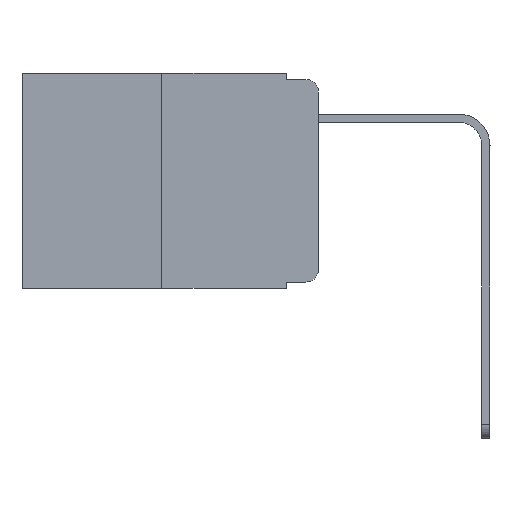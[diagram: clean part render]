
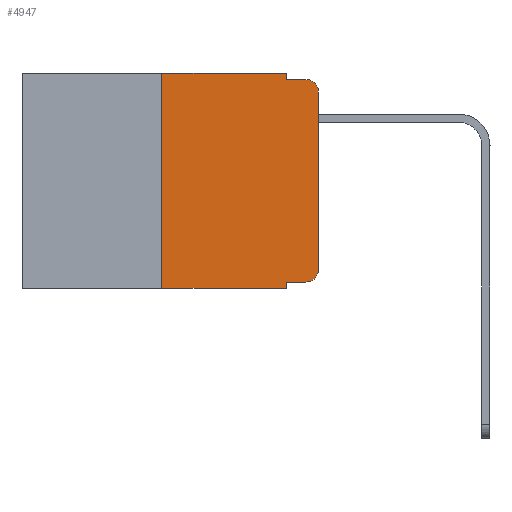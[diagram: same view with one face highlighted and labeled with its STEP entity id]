
A CAD part, left-side view. The second image highlights one B-rep face of the part: STEP entity #4947.
In plain terms, the highlighted planar face has unit normal (-1, 0, 0).
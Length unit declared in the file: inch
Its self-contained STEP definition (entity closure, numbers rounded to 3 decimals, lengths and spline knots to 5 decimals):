
#30 = VERTEX_POINT ( 'NONE', #19579 ) ;
#801 = CARTESIAN_POINT ( 'NONE',  ( 0., 0.051, -0.333 ) ) ;
#967 = ORIENTED_EDGE ( 'NONE', *, *, #7947, .F. ) ;
#1071 = VERTEX_POINT ( 'NONE', #11649 ) ;
#1330 = CARTESIAN_POINT ( 'NONE',  ( 0., 0., 0. ) ) ;
#1448 = AXIS2_PLACEMENT_3D ( 'NONE', #19015, #6102, #14162 ) ;
#1771 = VECTOR ( 'NONE', #10370, 39.37008 ) ;
#2011 = CARTESIAN_POINT ( 'NONE',  ( 0., 0.051, 0. ) ) ;
#2374 = VERTEX_POINT ( 'NONE', #12244 ) ;
#2958 = FACE_OUTER_BOUND ( 'NONE', #16848, .T. ) ;
#3194 = EDGE_CURVE ( 'NONE', #20260, #2374, #9029, .T. ) ;
#3876 = DIRECTION ( 'NONE',  ( 0., 0., -1. ) ) ;
#3958 = VECTOR ( 'NONE', #20413, 39.37008 ) ;
#4619 = ORIENTED_EDGE ( 'NONE', *, *, #20326, .T. ) ;
#4777 = DIRECTION ( 'NONE',  ( 0., 0., -1. ) ) ;
#4800 = DIRECTION ( 'NONE',  ( 0., -1., 0. ) ) ;
#4890 = LINE ( 'NONE', #6951, #16919 ) ;
#4947 = ADVANCED_FACE ( 'NONE', ( #2958 ), #19089, .F. ) ;
#5424 = VERTEX_POINT ( 'NONE', #17589 ) ;
#5590 = DIRECTION ( 'NONE',  ( 0., 0., 1. ) ) ;
#5600 = EDGE_CURVE ( 'NONE', #17703, #30, #14456, .T. ) ;
#6063 = CARTESIAN_POINT ( 'NONE',  ( 0., 0.02, -0.333 ) ) ;
#6102 = DIRECTION ( 'NONE',  ( -1., 0., 0. ) ) ;
#6338 = ORIENTED_EDGE ( 'NONE', *, *, #9061, .F. ) ;
#6361 = ORIENTED_EDGE ( 'NONE', *, *, #19386, .T. ) ;
#6453 = DIRECTION ( 'NONE',  ( 1., 0., 0. ) ) ;
#6568 = EDGE_CURVE ( 'NONE', #5424, #12130, #17664, .T. ) ;
#6638 = VERTEX_POINT ( 'NONE', #17126 ) ;
#6660 = DIRECTION ( 'NONE',  ( 0., 0., -1. ) ) ;
#6730 = DIRECTION ( 'NONE',  ( 0., -1., 0. ) ) ;
#6951 = CARTESIAN_POINT ( 'NONE',  ( 0., 0.051, -0.01 ) ) ;
#6972 = LINE ( 'NONE', #1330, #3958 ) ;
#6994 = CARTESIAN_POINT ( 'NONE',  ( 0., 0.051, 0. ) ) ;
#7091 = CARTESIAN_POINT ( 'NONE',  ( 0., 0.473, -0.343 ) ) ;
#7821 = VECTOR ( 'NONE', #6660, 39.37008 ) ;
#7947 = EDGE_CURVE ( 'NONE', #12130, #6638, #17270, .T. ) ;
#8411 = CARTESIAN_POINT ( 'NONE',  ( 0., 0.051, 0. ) ) ;
#8422 = VECTOR ( 'NONE', #20051, 39.37008 ) ;
#8543 = ORIENTED_EDGE ( 'NONE', *, *, #14179, .T. ) ;
#8610 = AXIS2_PLACEMENT_3D ( 'NONE', #11819, #11956, #3876 ) ;
#8659 = EDGE_CURVE ( 'NONE', #16283, #17703, #6972, .T. ) ;
#8861 = CARTESIAN_POINT ( 'NONE',  ( 0., 0.473, 0. ) ) ;
#9029 = LINE ( 'NONE', #8411, #7821 ) ;
#9061 = EDGE_CURVE ( 'NONE', #1071, #5424, #15926, .T. ) ;
#9890 = EDGE_CURVE ( 'NONE', #6638, #30, #4890, .T. ) ;
#10370 = DIRECTION ( 'NONE',  ( 0., -1., 0. ) ) ;
#11464 = ORIENTED_EDGE ( 'NONE', *, *, #6568, .F. ) ;
#11649 = CARTESIAN_POINT ( 'NONE',  ( 0., 0.25, -0.343 ) ) ;
#11819 = CARTESIAN_POINT ( 'NONE',  ( 0., 0.02, -0.313 ) ) ;
#11956 = DIRECTION ( 'NONE',  ( -1., 0., 0. ) ) ;
#12114 = CIRCLE ( 'NONE', #8610, 0.02 ) ;
#12130 = VERTEX_POINT ( 'NONE', #2011 ) ;
#12244 = CARTESIAN_POINT ( 'NONE',  ( 0., 0.051, -0.343 ) ) ;
#12806 = CARTESIAN_POINT ( 'NONE',  ( 0., 0.051, -0.333 ) ) ;
#12976 = LINE ( 'NONE', #7091, #1771 ) ;
#13326 = DIRECTION ( 'NONE',  ( 0., 0., -1. ) ) ;
#13751 = VECTOR ( 'NONE', #4800, 39.37008 ) ;
#13801 = VERTEX_POINT ( 'NONE', #6063 ) ;
#14162 = DIRECTION ( 'NONE',  ( 0., 0., -1. ) ) ;
#14179 = EDGE_CURVE ( 'NONE', #13801, #16283, #12114, .T. ) ;
#14456 = CIRCLE ( 'NONE', #1448, 0.02 ) ;
#14463 = CARTESIAN_POINT ( 'NONE',  ( 0., 0.473, 0. ) ) ;
#15133 = CARTESIAN_POINT ( 'NONE',  ( 0., 0.25, 0. ) ) ;
#15229 = VECTOR ( 'NONE', #13326, 39.37008 ) ;
#15775 = ORIENTED_EDGE ( 'NONE', *, *, #5600, .T. ) ;
#15926 = LINE ( 'NONE', #15133, #16455 ) ;
#16283 = VERTEX_POINT ( 'NONE', #17101 ) ;
#16455 = VECTOR ( 'NONE', #5590, 39.37008 ) ;
#16545 = LINE ( 'NONE', #12806, #13751 ) ;
#16848 = EDGE_LOOP ( 'NONE', ( #20553, #15775, #20427, #967, #11464, #6338, #4619, #17286, #6361, #8543 ) ) ;
#16919 = VECTOR ( 'NONE', #6730, 39.37008 ) ;
#16981 = AXIS2_PLACEMENT_3D ( 'NONE', #14463, #6453, #4777 ) ;
#17101 = CARTESIAN_POINT ( 'NONE',  ( 0., 0., -0.313 ) ) ;
#17126 = CARTESIAN_POINT ( 'NONE',  ( 0., 0.051, -0.01 ) ) ;
#17270 = LINE ( 'NONE', #6994, #15229 ) ;
#17286 = ORIENTED_EDGE ( 'NONE', *, *, #3194, .F. ) ;
#17589 = CARTESIAN_POINT ( 'NONE',  ( 0., 0.25, 0. ) ) ;
#17664 = LINE ( 'NONE', #8861, #8422 ) ;
#17703 = VERTEX_POINT ( 'NONE', #17935 ) ;
#17935 = CARTESIAN_POINT ( 'NONE',  ( 0., 0., -0.03 ) ) ;
#19015 = CARTESIAN_POINT ( 'NONE',  ( 0., 0.02, -0.03 ) ) ;
#19089 = PLANE ( 'NONE',  #16981 ) ;
#19386 = EDGE_CURVE ( 'NONE', #20260, #13801, #16545, .T. ) ;
#19579 = CARTESIAN_POINT ( 'NONE',  ( 0., 0.02, -0.01 ) ) ;
#20051 = DIRECTION ( 'NONE',  ( 0., -1., 0. ) ) ;
#20260 = VERTEX_POINT ( 'NONE', #801 ) ;
#20326 = EDGE_CURVE ( 'NONE', #1071, #2374, #12976, .T. ) ;
#20413 = DIRECTION ( 'NONE',  ( 0., 0., 1. ) ) ;
#20427 = ORIENTED_EDGE ( 'NONE', *, *, #9890, .F. ) ;
#20553 = ORIENTED_EDGE ( 'NONE', *, *, #8659, .T. ) ;
